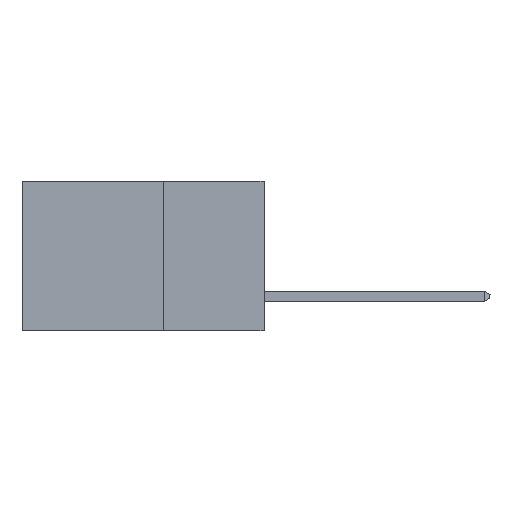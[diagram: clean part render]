
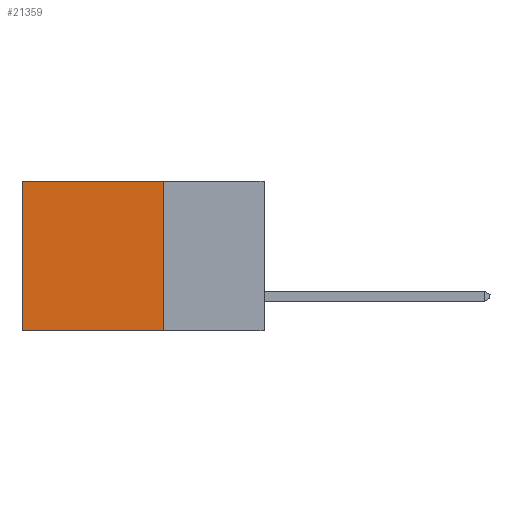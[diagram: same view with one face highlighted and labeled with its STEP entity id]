
A CAD part, left-side view. The second image highlights one B-rep face of the part: STEP entity #21359.
In plain terms, the highlighted planar face has unit normal (-1, 0, 0).
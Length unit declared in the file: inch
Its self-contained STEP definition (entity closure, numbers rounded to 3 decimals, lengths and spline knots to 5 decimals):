
#218 = VECTOR ( 'NONE', #15200, 39.37008 ) ;
#1442 = CARTESIAN_POINT ( 'NONE',  ( 0.298, 0.25, 0. ) ) ;
#1832 = PLANE ( 'NONE',  #21735 ) ;
#1841 = CARTESIAN_POINT ( 'NONE',  ( 0.298, 0.6, 0. ) ) ;
#2506 = ORIENTED_EDGE ( 'NONE', *, *, #19586, .F. ) ;
#3280 = DIRECTION ( 'NONE',  ( 0., 1., 0. ) ) ;
#4222 = LINE ( 'NONE', #11239, #218 ) ;
#4355 = ORIENTED_EDGE ( 'NONE', *, *, #5701, .T. ) ;
#5151 = ORIENTED_EDGE ( 'NONE', *, *, #19030, .T. ) ;
#5382 = VERTEX_POINT ( 'NONE', #1841 ) ;
#5701 = EDGE_CURVE ( 'NONE', #11218, #5382, #15179, .T. ) ;
#6651 = EDGE_LOOP ( 'NONE', ( #5151, #2506, #7861, #4355 ) ) ;
#7141 = LINE ( 'NONE', #20313, #11209 ) ;
#7350 = DIRECTION ( 'NONE',  ( 0., 1., 0. ) ) ;
#7660 = EDGE_CURVE ( 'NONE', #11218, #17529, #7141, .T. ) ;
#7861 = ORIENTED_EDGE ( 'NONE', *, *, #7660, .F. ) ;
#8117 = FACE_OUTER_BOUND ( 'NONE', #6651, .T. ) ;
#11209 = VECTOR ( 'NONE', #14206, 39.37008 ) ;
#11218 = VERTEX_POINT ( 'NONE', #1442 ) ;
#11239 = CARTESIAN_POINT ( 'NONE',  ( 0.298, 0.6, 0. ) ) ;
#14206 = DIRECTION ( 'NONE',  ( 0., 0., -1. ) ) ;
#15179 = LINE ( 'NONE', #25386, #16115 ) ;
#15200 = DIRECTION ( 'NONE',  ( 0., 0., -1. ) ) ;
#15874 = CARTESIAN_POINT ( 'NONE',  ( 0.298, 0.25, 0. ) ) ;
#16115 = VECTOR ( 'NONE', #3280, 39.37008 ) ;
#17529 = VERTEX_POINT ( 'NONE', #24156 ) ;
#17943 = DIRECTION ( 'NONE',  ( 0., 0., -1. ) ) ;
#19030 = EDGE_CURVE ( 'NONE', #5382, #23920, #4222, .T. ) ;
#19275 = CARTESIAN_POINT ( 'NONE',  ( 0.298, 0.6, -0.37 ) ) ;
#19586 = EDGE_CURVE ( 'NONE', #17529, #23920, #24372, .T. ) ;
#20313 = CARTESIAN_POINT ( 'NONE',  ( 0.298, 0.25, 0. ) ) ;
#21359 = ADVANCED_FACE ( 'NONE', ( #8117 ), #1832, .F. ) ;
#21486 = CARTESIAN_POINT ( 'NONE',  ( 0.298, 0.25, -0.37 ) ) ;
#21735 = AXIS2_PLACEMENT_3D ( 'NONE', #15874, #23763, #17943 ) ;
#22477 = VECTOR ( 'NONE', #7350, 39.37008 ) ;
#23763 = DIRECTION ( 'NONE',  ( 1., 0., 0. ) ) ;
#23920 = VERTEX_POINT ( 'NONE', #19275 ) ;
#24156 = CARTESIAN_POINT ( 'NONE',  ( 0.298, 0.25, -0.37 ) ) ;
#24372 = LINE ( 'NONE', #21486, #22477 ) ;
#25386 = CARTESIAN_POINT ( 'NONE',  ( 0.298, 0.25, 0. ) ) ;
